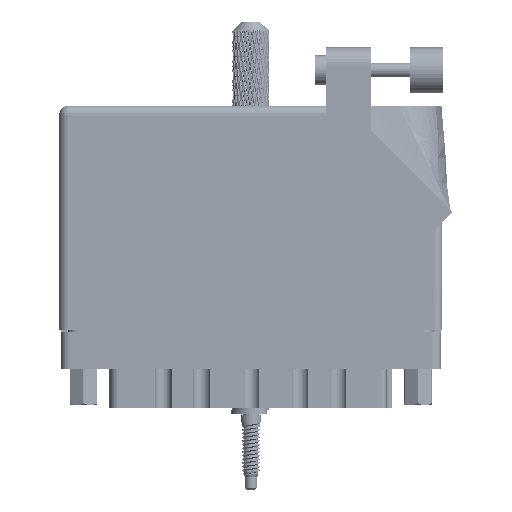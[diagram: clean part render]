
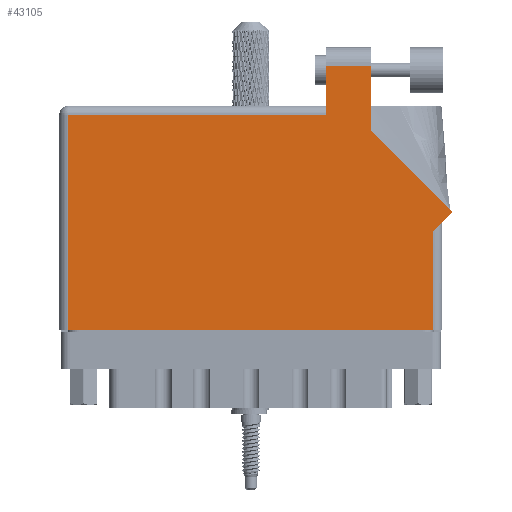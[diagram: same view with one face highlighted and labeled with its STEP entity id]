
A CAD part, front view. The second image highlights one B-rep face of the part: STEP entity #43105.
In plain terms, the highlighted face is planar.
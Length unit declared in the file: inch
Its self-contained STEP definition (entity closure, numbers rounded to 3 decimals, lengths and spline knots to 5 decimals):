
#1467 = ORIENTED_EDGE ( 'NONE', *, *, #25204, .T. ) ;
#6625 = VECTOR ( 'NONE', #26599, 39.37008 ) ;
#6686 = CARTESIAN_POINT ( 'NONE',  ( 2.68271, 0.80771, 0. ) ) ;
#7378 = CARTESIAN_POINT ( 'NONE',  ( 1.819, 1.805, 0. ) ) ;
#7422 = EDGE_CURVE ( 'NONE', #117987, #78943, #82945, .T. ) ;
#9135 = DIRECTION ( 'NONE',  ( -1., 0., 0. ) ) ;
#9720 = LINE ( 'NONE', #6686, #6625 ) ;
#9931 = VECTOR ( 'NONE', #84509, 39.37008 ) ;
#11437 = LINE ( 'NONE', #17081, #9931 ) ;
#11620 = LINE ( 'NONE', #48349, #28649 ) ;
#14987 = ORIENTED_EDGE ( 'NONE', *, *, #85402, .T. ) ;
#15850 = EDGE_CURVE ( 'NONE', #116926, #101379, #49468, .T. ) ;
#16566 = DIRECTION ( 'NONE',  ( 0.707, 0.707, 0. ) ) ;
#16836 = LINE ( 'NONE', #18560, #120508 ) ;
#17081 = CARTESIAN_POINT ( 'NONE',  ( 0.062, 0., 0. ) ) ;
#18560 = CARTESIAN_POINT ( 'NONE',  ( 1.819, 1.53, 0. ) ) ;
#18963 = EDGE_CURVE ( 'NONE', #70886, #55162, #79897, .T. ) ;
#19062 = CARTESIAN_POINT ( 'NONE',  ( 0., 1.53, 0. ) ) ;
#24662 = VECTOR ( 'NONE', #95536, 39.37008 ) ;
#25204 = EDGE_CURVE ( 'NONE', #101379, #49605, #103642, .T. ) ;
#26599 = DIRECTION ( 'NONE',  ( -0.707, 0.707, 0. ) ) ;
#28649 = VECTOR ( 'NONE', #88086, 39.37008 ) ;
#29834 = CARTESIAN_POINT ( 'NONE',  ( 1.819, 1.468, 0. ) ) ;
#29970 = ORIENTED_EDGE ( 'NONE', *, *, #71277, .T. ) ;
#30331 = AXIS2_PLACEMENT_3D ( 'NONE', #19062, #108147, #9135 ) ;
#32920 = EDGE_CURVE ( 'NONE', #49605, #87516, #16836, .T. ) ;
#35713 = ORIENTED_EDGE ( 'NONE', *, *, #7422, .T. ) ;
#36141 = CARTESIAN_POINT ( 'NONE',  ( 2.126, 1.36442, 0. ) ) ;
#38735 = CARTESIAN_POINT ( 'NONE',  ( 2.126, 1.805, 0. ) ) ;
#38738 = EDGE_LOOP ( 'NONE', ( #89061, #1467, #52584, #14987, #29970, #75526, #98349, #35713, #76874 ) ) ;
#43105 = ADVANCED_FACE ( 'NONE', ( #82162 ), #108582, .F. ) ;
#48349 = CARTESIAN_POINT ( 'NONE',  ( 2.55, 0.737, 0. ) ) ;
#49468 = LINE ( 'NONE', #85603, #24662 ) ;
#49605 = VERTEX_POINT ( 'NONE', #75278 ) ;
#50459 = VECTOR ( 'NONE', #16566, 39.37008 ) ;
#52584 = ORIENTED_EDGE ( 'NONE', *, *, #32920, .T. ) ;
#55162 = VERTEX_POINT ( 'NONE', #111962 ) ;
#70886 = VERTEX_POINT ( 'NONE', #73837 ) ;
#71277 = EDGE_CURVE ( 'NONE', #100305, #70886, #11437, .T. ) ;
#71925 = CARTESIAN_POINT ( 'NONE',  ( 0., 1.468, 0. ) ) ;
#73837 = CARTESIAN_POINT ( 'NONE',  ( 0.062, 0., 0. ) ) ;
#75278 = CARTESIAN_POINT ( 'NONE',  ( 1.819, 1.805, 0. ) ) ;
#75526 = ORIENTED_EDGE ( 'NONE', *, *, #18963, .T. ) ;
#76874 = ORIENTED_EDGE ( 'NONE', *, *, #100046, .T. ) ;
#78515 = VECTOR ( 'NONE', #121691, 39.37008 ) ;
#78943 = VERTEX_POINT ( 'NONE', #84028 ) ;
#79897 = LINE ( 'NONE', #119049, #104696 ) ;
#82162 = FACE_OUTER_BOUND ( 'NONE', #38738, .T. ) ;
#82945 = LINE ( 'NONE', #95661, #50459 ) ;
#84028 = CARTESIAN_POINT ( 'NONE',  ( 2.68271, 0.80771, 0. ) ) ;
#84509 = DIRECTION ( 'NONE',  ( 0., -1., 0. ) ) ;
#85402 = EDGE_CURVE ( 'NONE', #87516, #100305, #117408, .T. ) ;
#85603 = CARTESIAN_POINT ( 'NONE',  ( 2.126, 1.36442, 0. ) ) ;
#86471 = DIRECTION ( 'NONE',  ( -1., 0., 0. ) ) ;
#87516 = VERTEX_POINT ( 'NONE', #29834 ) ;
#87712 = DIRECTION ( 'NONE',  ( 0., -1., 0. ) ) ;
#88086 = DIRECTION ( 'NONE',  ( 0., 1., 0. ) ) ;
#88410 = EDGE_CURVE ( 'NONE', #55162, #117987, #11620, .T. ) ;
#89061 = ORIENTED_EDGE ( 'NONE', *, *, #15850, .T. ) ;
#95209 = CARTESIAN_POINT ( 'NONE',  ( 2.55, 0.675, 0. ) ) ;
#95536 = DIRECTION ( 'NONE',  ( 0., 1., 0. ) ) ;
#95661 = CARTESIAN_POINT ( 'NONE',  ( 2.612, 0.737, 0. ) ) ;
#98349 = ORIENTED_EDGE ( 'NONE', *, *, #88410, .T. ) ;
#100046 = EDGE_CURVE ( 'NONE', #78943, #116926, #9720, .T. ) ;
#100305 = VERTEX_POINT ( 'NONE', #121233 ) ;
#101379 = VERTEX_POINT ( 'NONE', #38735 ) ;
#101924 = DIRECTION ( 'NONE',  ( 1., 0., 0. ) ) ;
#103642 = LINE ( 'NONE', #7378, #126977 ) ;
#104696 = VECTOR ( 'NONE', #101924, 39.37008 ) ;
#108147 = DIRECTION ( 'NONE',  ( 0., 0., -1. ) ) ;
#108582 = PLANE ( 'NONE',  #30331 ) ;
#111962 = CARTESIAN_POINT ( 'NONE',  ( 2.55, 0., 0. ) ) ;
#116926 = VERTEX_POINT ( 'NONE', #36141 ) ;
#117408 = LINE ( 'NONE', #71925, #78515 ) ;
#117987 = VERTEX_POINT ( 'NONE', #95209 ) ;
#119049 = CARTESIAN_POINT ( 'NONE',  ( 0., 0., 0. ) ) ;
#120508 = VECTOR ( 'NONE', #87712, 39.37008 ) ;
#121233 = CARTESIAN_POINT ( 'NONE',  ( 0.062, 1.468, 0. ) ) ;
#121691 = DIRECTION ( 'NONE',  ( -1., 0., 0. ) ) ;
#126977 = VECTOR ( 'NONE', #86471, 39.37008 ) ;
